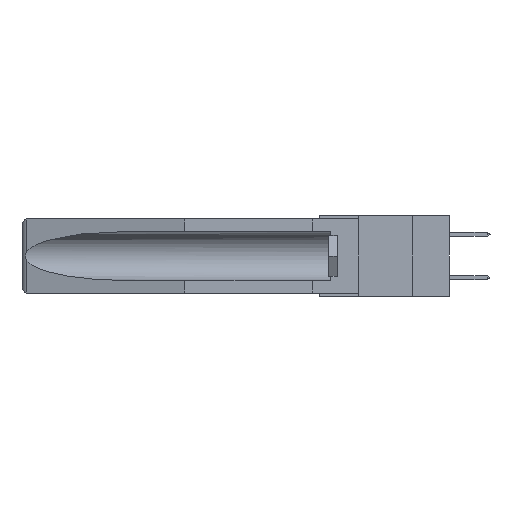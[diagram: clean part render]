
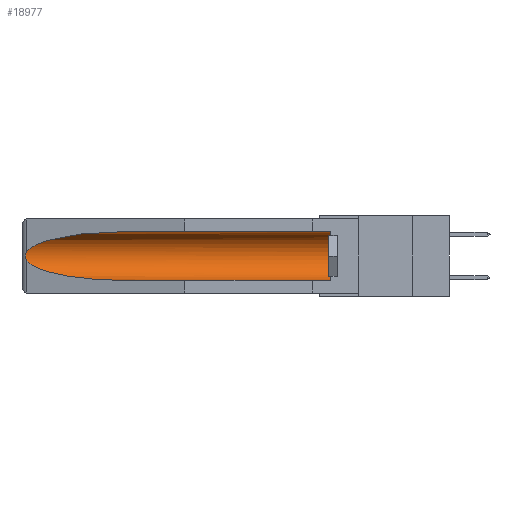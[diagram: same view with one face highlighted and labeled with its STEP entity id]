
A CAD part, left-side view. The second image highlights one B-rep face of the part: STEP entity #18977.
In plain terms, the highlighted cylindrical face has radius 2.857 mm (diameter 5.715 mm), a partial arc.
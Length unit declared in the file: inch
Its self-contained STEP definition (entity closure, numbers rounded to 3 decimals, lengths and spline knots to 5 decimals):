
#59 = EDGE_CURVE ( 'NONE', #27776, #24340, #18574, .T. ) ;
#63 = DIRECTION ( 'NONE',  ( 0., 0., 1. ) ) ;
#422 =( BOUNDED_CURVE ( )  B_SPLINE_CURVE ( 3, ( #30334, #1625, #19276, #4144 ),
 .UNSPECIFIED., .F., .F. ) 
 B_SPLINE_CURVE_WITH_KNOTS ( ( 4, 4 ),
 ( 0.1948, 1.5708 ),
 .UNSPECIFIED. ) 
 CURVE ( )  GEOMETRIC_REPRESENTATION_ITEM ( )  RATIONAL_B_SPLINE_CURVE ( ( 1., 0.848, 0.848, 1. ) ) 
 REPRESENTATION_ITEM ( '' )  );
#1625 = CARTESIAN_POINT ( 'NONE',  ( 0.25451, 1.48313, -0.24835 ) ) ;
#2044 = CARTESIAN_POINT ( 'NONE',  ( 0.155, -0.30754, -0.1715 ) ) ;
#2809 = EDGE_LOOP ( 'NONE', ( #14740, #30877, #23484, #6063, #21130, #16263 ) ) ;
#4073 = EDGE_CURVE ( 'NONE', #4484, #25687, #23806, .T. ) ;
#4144 = CARTESIAN_POINT ( 'NONE',  ( 0.155, 1.07973, -0.284 ) ) ;
#4484 = VERTEX_POINT ( 'NONE', #32503 ) ;
#4485 = CARTESIAN_POINT ( 'NONE',  ( 0.155, 0.126, -0.059 ) ) ;
#5242 = VECTOR ( 'NONE', #6514, 39.37008 ) ;
#5408 = DIRECTION ( 'NONE',  ( 0., 1., 0. ) ) ;
#5565 = CARTESIAN_POINT ( 'NONE',  ( 0.155, 1.07973, -0.059 ) ) ;
#5893 = AXIS2_PLACEMENT_3D ( 'NONE', #20112, #7302, #63 ) ;
#6063 = ORIENTED_EDGE ( 'NONE', *, *, #4073, .F. ) ;
#6514 = DIRECTION ( 'NONE',  ( 0., 1., 0. ) ) ;
#6948 = CARTESIAN_POINT ( 'NONE',  ( 0.26654, 1.53092, -0.15636 ) ) ;
#7302 = DIRECTION ( 'NONE',  ( 0., -1., 0. ) ) ;
#8451 = CARTESIAN_POINT ( 'NONE',  ( 0.26537, 1.52718, -0.19328 ) ) ;
#8877 = CARTESIAN_POINT ( 'NONE',  ( 0.155, 1.07973, -0.284 ) ) ;
#9269 = CIRCLE ( 'NONE', #5893, 0.1125 ) ;
#10418 = VERTEX_POINT ( 'NONE', #17205 ) ;
#11411 = CARTESIAN_POINT ( 'NONE',  ( 0.155, -0.30754, -0.284 ) ) ;
#12384 = CARTESIAN_POINT ( 'NONE',  ( 0.26537, 1.52718, -0.14972 ) ) ;
#13083 = DIRECTION ( 'NONE',  ( 0., 0., 1. ) ) ;
#14681 = CARTESIAN_POINT ( 'NONE',  ( 0.2675, 1.53308, -0.16763 ) ) ;
#14740 = ORIENTED_EDGE ( 'NONE', *, *, #18469, .T. ) ;
#14907 = CARTESIAN_POINT ( 'NONE',  ( 0.26537, 1.52718, -0.19328 ) ) ;
#16263 = ORIENTED_EDGE ( 'NONE', *, *, #59, .T. ) ;
#17205 = CARTESIAN_POINT ( 'NONE',  ( 0.26537, 1.52718, -0.14972 ) ) ;
#17236 = CARTESIAN_POINT ( 'NONE',  ( 0.26597, 1.52961, -0.15275 ) ) ;
#17988 = CARTESIAN_POINT ( 'NONE',  ( 0.155, -0.30754, -0.059 ) ) ;
#18386 = EDGE_CURVE ( 'NONE', #32593, #25687, #422, .T. ) ;
#18469 = EDGE_CURVE ( 'NONE', #24340, #10418, #25477, .T. ) ;
#18574 = LINE ( 'NONE', #17988, #23298 ) ;
#18627 = B_SPLINE_CURVE_WITH_KNOTS ( 'NONE', 3,
 ( #12384, #17236, #6948, #19743, #14681, #30066, #24941, #27620, #32260, #14907 ),
 .UNSPECIFIED., .F., .F.,
 ( 4, 2, 2, 2, 4 ),
 ( 0., 0.00029, 0.00058, 0.00087, 0.00117 ),
 .UNSPECIFIED. ) ;
#18977 = ADVANCED_FACE ( 'NONE', ( #22568 ), #25336, .F. ) ;
#19276 = CARTESIAN_POINT ( 'NONE',  ( 0.21114, 1.30732, -0.284 ) ) ;
#19743 = CARTESIAN_POINT ( 'NONE',  ( 0.2673, 1.5327, -0.16383 ) ) ;
#20112 = CARTESIAN_POINT ( 'NONE',  ( 0.155, 0.126, -0.1715 ) ) ;
#21130 = ORIENTED_EDGE ( 'NONE', *, *, #31133, .T. ) ;
#21948 = AXIS2_PLACEMENT_3D ( 'NONE', #2044, #22210, #13083 ) ;
#22210 = DIRECTION ( 'NONE',  ( 0., 1., 0. ) ) ;
#22330 = CARTESIAN_POINT ( 'NONE',  ( 0.155, 1.07973, -0.059 ) ) ;
#22568 = FACE_OUTER_BOUND ( 'NONE', #2809, .T. ) ;
#23206 = CARTESIAN_POINT ( 'NONE',  ( 0.21114, 1.30732, -0.059 ) ) ;
#23298 = VECTOR ( 'NONE', #5408, 39.37008 ) ;
#23484 = ORIENTED_EDGE ( 'NONE', *, *, #18386, .T. ) ;
#23806 = LINE ( 'NONE', #11411, #5242 ) ;
#24340 = VERTEX_POINT ( 'NONE', #22330 ) ;
#24941 = CARTESIAN_POINT ( 'NONE',  ( 0.2673, 1.53269, -0.17917 ) ) ;
#25314 = CARTESIAN_POINT ( 'NONE',  ( 0.25451, 1.48313, -0.09465 ) ) ;
#25336 = CYLINDRICAL_SURFACE ( 'NONE', #21948, 0.1125 ) ;
#25477 =( BOUNDED_CURVE ( )  B_SPLINE_CURVE ( 3, ( #5565, #23206, #25314, #27885 ),
 .UNSPECIFIED., .F., .F. ) 
 B_SPLINE_CURVE_WITH_KNOTS ( ( 4, 4 ),
 ( 4.71239, 6.08839 ),
 .UNSPECIFIED. ) 
 CURVE ( )  GEOMETRIC_REPRESENTATION_ITEM ( )  RATIONAL_B_SPLINE_CURVE ( ( 1., 0.848, 0.848, 1. ) ) 
 REPRESENTATION_ITEM ( '' )  );
#25687 = VERTEX_POINT ( 'NONE', #8877 ) ;
#27620 = CARTESIAN_POINT ( 'NONE',  ( 0.26655, 1.53094, -0.18657 ) ) ;
#27776 = VERTEX_POINT ( 'NONE', #4485 ) ;
#27885 = CARTESIAN_POINT ( 'NONE',  ( 0.26537, 1.52718, -0.14972 ) ) ;
#28961 = EDGE_CURVE ( 'NONE', #10418, #32593, #18627, .T. ) ;
#30066 = CARTESIAN_POINT ( 'NONE',  ( 0.2675, 1.53308, -0.17534 ) ) ;
#30334 = CARTESIAN_POINT ( 'NONE',  ( 0.26537, 1.52718, -0.19328 ) ) ;
#30877 = ORIENTED_EDGE ( 'NONE', *, *, #28961, .T. ) ;
#31133 = EDGE_CURVE ( 'NONE', #4484, #27776, #9269, .T. ) ;
#32260 = CARTESIAN_POINT ( 'NONE',  ( 0.26597, 1.5296, -0.19026 ) ) ;
#32503 = CARTESIAN_POINT ( 'NONE',  ( 0.155, 0.126, -0.284 ) ) ;
#32593 = VERTEX_POINT ( 'NONE', #8451 ) ;
